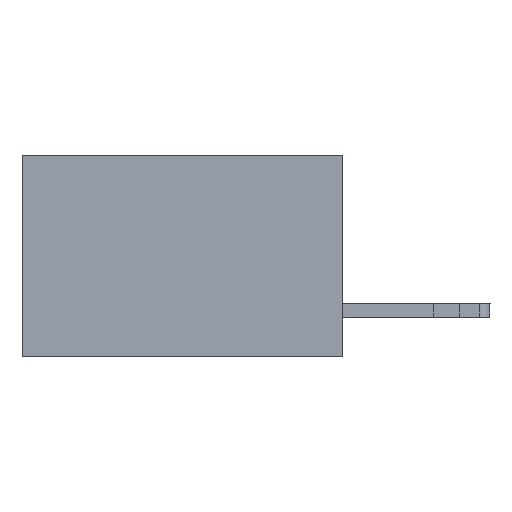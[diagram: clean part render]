
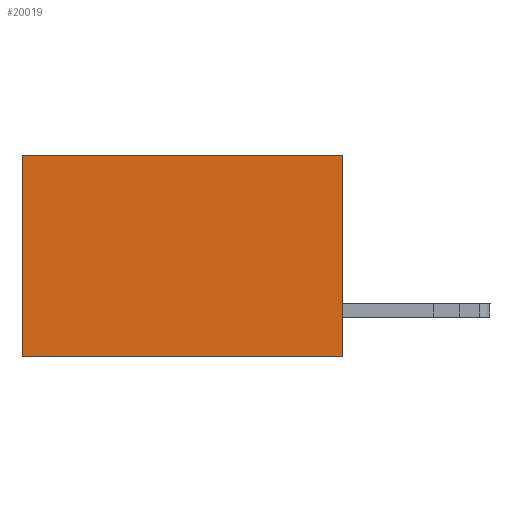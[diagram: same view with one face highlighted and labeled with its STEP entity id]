
A CAD part, left-side view. The second image highlights one B-rep face of the part: STEP entity #20019.
In plain terms, the highlighted planar face has unit normal (-1, 0, 0).
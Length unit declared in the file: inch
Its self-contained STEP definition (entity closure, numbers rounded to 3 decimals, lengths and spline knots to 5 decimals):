
#804 = EDGE_CURVE ( 'NONE', #11876, #2926, #13203, .T. ) ;
#1502 = DIRECTION ( 'NONE',  ( 0., 0., -1. ) ) ;
#2838 = LINE ( 'NONE', #23554, #12409 ) ;
#2926 = VERTEX_POINT ( 'NONE', #17847 ) ;
#4302 = VECTOR ( 'NONE', #15747, 39.37008 ) ;
#4822 = AXIS2_PLACEMENT_3D ( 'NONE', #21680, #10799, #23523 ) ;
#5384 = LINE ( 'NONE', #17663, #14744 ) ;
#6134 = ORIENTED_EDGE ( 'NONE', *, *, #804, .F. ) ;
#6532 = VECTOR ( 'NONE', #1502, 39.37008 ) ;
#8847 = EDGE_CURVE ( 'NONE', #17281, #11555, #5384, .T. ) ;
#8909 = PLANE ( 'NONE',  #4822 ) ;
#10065 = EDGE_CURVE ( 'NONE', #11555, #2926, #16368, .T. ) ;
#10799 = DIRECTION ( 'NONE',  ( 1., 0., 0. ) ) ;
#10895 = CARTESIAN_POINT ( 'NONE',  ( 0.277, 0., 0. ) ) ;
#11409 = CARTESIAN_POINT ( 'NONE',  ( 0.277, 0., -0.37 ) ) ;
#11555 = VERTEX_POINT ( 'NONE', #13372 ) ;
#11876 = VERTEX_POINT ( 'NONE', #12724 ) ;
#12409 = VECTOR ( 'NONE', #19868, 39.37008 ) ;
#12724 = CARTESIAN_POINT ( 'NONE',  ( 0.277, 0., -0.37 ) ) ;
#13203 = LINE ( 'NONE', #11409, #4302 ) ;
#13310 = ORIENTED_EDGE ( 'NONE', *, *, #10065, .T. ) ;
#13372 = CARTESIAN_POINT ( 'NONE',  ( 0.277, 0.59, 0. ) ) ;
#14744 = VECTOR ( 'NONE', #21306, 39.37008 ) ;
#15747 = DIRECTION ( 'NONE',  ( 0., 1., 0. ) ) ;
#16368 = LINE ( 'NONE', #18333, #6532 ) ;
#16624 = EDGE_LOOP ( 'NONE', ( #13310, #6134, #23447, #22614 ) ) ;
#17281 = VERTEX_POINT ( 'NONE', #10895 ) ;
#17663 = CARTESIAN_POINT ( 'NONE',  ( 0.277, 0., 0. ) ) ;
#17847 = CARTESIAN_POINT ( 'NONE',  ( 0.277, 0.59, -0.37 ) ) ;
#18333 = CARTESIAN_POINT ( 'NONE',  ( 0.277, 0.59, -0.37 ) ) ;
#19371 = EDGE_CURVE ( 'NONE', #17281, #11876, #2838, .T. ) ;
#19868 = DIRECTION ( 'NONE',  ( 0., 0., -1. ) ) ;
#20019 = ADVANCED_FACE ( 'NONE', ( #21173 ), #8909, .F. ) ;
#21173 = FACE_OUTER_BOUND ( 'NONE', #16624, .T. ) ;
#21306 = DIRECTION ( 'NONE',  ( 0., 1., 0. ) ) ;
#21680 = CARTESIAN_POINT ( 'NONE',  ( 0.277, 0., -0.37 ) ) ;
#22614 = ORIENTED_EDGE ( 'NONE', *, *, #8847, .T. ) ;
#23447 = ORIENTED_EDGE ( 'NONE', *, *, #19371, .F. ) ;
#23523 = DIRECTION ( 'NONE',  ( 0., 0., -1. ) ) ;
#23554 = CARTESIAN_POINT ( 'NONE',  ( 0.277, 0., -0.37 ) ) ;
